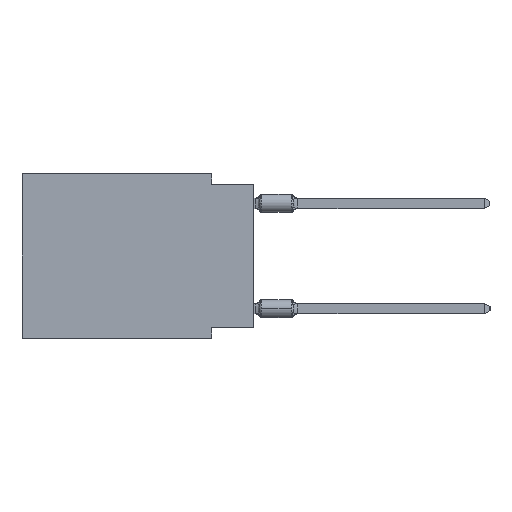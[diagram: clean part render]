
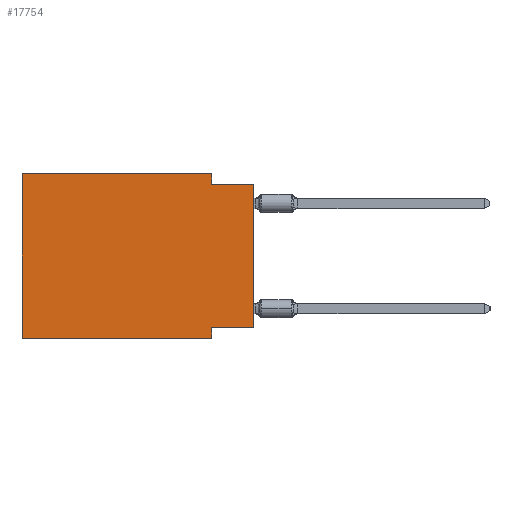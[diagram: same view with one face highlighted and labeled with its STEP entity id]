
A CAD part, left-side view. The second image highlights one B-rep face of the part: STEP entity #17754.
In plain terms, the highlighted planar face has unit normal (-1, 0, 0).
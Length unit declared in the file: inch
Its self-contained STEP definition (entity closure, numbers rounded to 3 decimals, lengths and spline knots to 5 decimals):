
#458 = ORIENTED_EDGE ( 'NONE', *, *, #26284, .F. ) ;
#755 = ORIENTED_EDGE ( 'NONE', *, *, #5786, .F. ) ;
#885 = LINE ( 'NONE', #16371, #30595 ) ;
#900 = LINE ( 'NONE', #11897, #17409 ) ;
#985 = VECTOR ( 'NONE', #10773, 39.37008 ) ;
#1927 = CARTESIAN_POINT ( 'NONE',  ( 0., 0.1, -0.025 ) ) ;
#3042 = VERTEX_POINT ( 'NONE', #17719 ) ;
#3174 = VECTOR ( 'NONE', #30415, 39.37008 ) ;
#4197 = ORIENTED_EDGE ( 'NONE', *, *, #18093, .F. ) ;
#5786 = EDGE_CURVE ( 'NONE', #14091, #29681, #9490, .T. ) ;
#6526 = CARTESIAN_POINT ( 'NONE',  ( 0., 0., -0.365 ) ) ;
#6831 = EDGE_CURVE ( 'NONE', #14091, #12727, #900, .T. ) ;
#9066 = DIRECTION ( 'NONE',  ( 0., -1., 0. ) ) ;
#9399 = LINE ( 'NONE', #20231, #29694 ) ;
#9490 = LINE ( 'NONE', #23364, #26731 ) ;
#10266 = EDGE_CURVE ( 'NONE', #30679, #32193, #9399, .T. ) ;
#10311 = DIRECTION ( 'NONE',  ( 0., 0., 1. ) ) ;
#10773 = DIRECTION ( 'NONE',  ( 0., 0., -1. ) ) ;
#11897 = CARTESIAN_POINT ( 'NONE',  ( 0., 0.55, -0.39 ) ) ;
#12001 = CARTESIAN_POINT ( 'NONE',  ( 0., 0.1, -0.39 ) ) ;
#12285 = CARTESIAN_POINT ( 'NONE',  ( 0., 0.55, 0. ) ) ;
#12727 = VERTEX_POINT ( 'NONE', #12001 ) ;
#13193 = ORIENTED_EDGE ( 'NONE', *, *, #16290, .F. ) ;
#13846 = CARTESIAN_POINT ( 'NONE',  ( 0., 0.1, -0.39 ) ) ;
#14091 = VERTEX_POINT ( 'NONE', #20944 ) ;
#14375 = ORIENTED_EDGE ( 'NONE', *, *, #6831, .T. ) ;
#15581 = CARTESIAN_POINT ( 'NONE',  ( 0., 0.1, 0. ) ) ;
#16290 = EDGE_CURVE ( 'NONE', #28372, #30679, #18332, .T. ) ;
#16371 = CARTESIAN_POINT ( 'NONE',  ( 0., 0., 0. ) ) ;
#17409 = VECTOR ( 'NONE', #27055, 39.37008 ) ;
#17719 = CARTESIAN_POINT ( 'NONE',  ( 0., 0., -0.365 ) ) ;
#17754 = ADVANCED_FACE ( 'NONE', ( #30698 ), #25357, .F. ) ;
#18093 = EDGE_CURVE ( 'NONE', #3042, #20592, #24583, .T. ) ;
#18332 = LINE ( 'NONE', #15581, #985 ) ;
#19845 = VECTOR ( 'NONE', #25786, 39.37008 ) ;
#20231 = CARTESIAN_POINT ( 'NONE',  ( 0., 0., -0.025 ) ) ;
#20592 = VERTEX_POINT ( 'NONE', #22386 ) ;
#20797 = ORIENTED_EDGE ( 'NONE', *, *, #24567, .T. ) ;
#20944 = CARTESIAN_POINT ( 'NONE',  ( 0., 0.55, -0.39 ) ) ;
#20966 = LINE ( 'NONE', #30954, #19845 ) ;
#22296 = CARTESIAN_POINT ( 'NONE',  ( 0., 0.1, 0. ) ) ;
#22386 = CARTESIAN_POINT ( 'NONE',  ( 0., 0.1, -0.365 ) ) ;
#22770 = DIRECTION ( 'NONE',  ( 1., 0., 0. ) ) ;
#23199 = ORIENTED_EDGE ( 'NONE', *, *, #10266, .F. ) ;
#23364 = CARTESIAN_POINT ( 'NONE',  ( 0., 0.55, 0. ) ) ;
#24282 = DIRECTION ( 'NONE',  ( 0., 0., 1. ) ) ;
#24567 = EDGE_CURVE ( 'NONE', #3042, #32193, #885, .T. ) ;
#24583 = LINE ( 'NONE', #6526, #3174 ) ;
#25357 = PLANE ( 'NONE',  #29506 ) ;
#25786 = DIRECTION ( 'NONE',  ( 0., -1., 0. ) ) ;
#25834 = ORIENTED_EDGE ( 'NONE', *, *, #32218, .F. ) ;
#26284 = EDGE_CURVE ( 'NONE', #20592, #12727, #33206, .T. ) ;
#26299 = CARTESIAN_POINT ( 'NONE',  ( 0., 0., -0.025 ) ) ;
#26731 = VECTOR ( 'NONE', #10311, 39.37008 ) ;
#27055 = DIRECTION ( 'NONE',  ( 0., -1., 0. ) ) ;
#27680 = CARTESIAN_POINT ( 'NONE',  ( 0., 0.55, 0. ) ) ;
#28372 = VERTEX_POINT ( 'NONE', #22296 ) ;
#29506 = AXIS2_PLACEMENT_3D ( 'NONE', #12285, #22770, #33265 ) ;
#29681 = VERTEX_POINT ( 'NONE', #27680 ) ;
#29694 = VECTOR ( 'NONE', #9066, 39.37008 ) ;
#30238 = EDGE_LOOP ( 'NONE', ( #20797, #23199, #13193, #25834, #755, #14375, #458, #4197 ) ) ;
#30415 = DIRECTION ( 'NONE',  ( 0., 1., 0. ) ) ;
#30458 = DIRECTION ( 'NONE',  ( 0., 0., -1. ) ) ;
#30595 = VECTOR ( 'NONE', #24282, 39.37008 ) ;
#30679 = VERTEX_POINT ( 'NONE', #1927 ) ;
#30698 = FACE_OUTER_BOUND ( 'NONE', #30238, .T. ) ;
#30954 = CARTESIAN_POINT ( 'NONE',  ( 0., 0.55, 0. ) ) ;
#32193 = VERTEX_POINT ( 'NONE', #26299 ) ;
#32218 = EDGE_CURVE ( 'NONE', #29681, #28372, #20966, .T. ) ;
#32846 = VECTOR ( 'NONE', #30458, 39.37008 ) ;
#33206 = LINE ( 'NONE', #13846, #32846 ) ;
#33265 = DIRECTION ( 'NONE',  ( 0., 0., -1. ) ) ;
